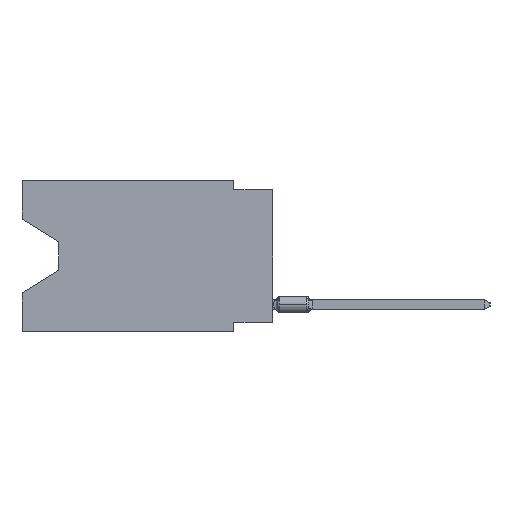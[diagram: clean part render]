
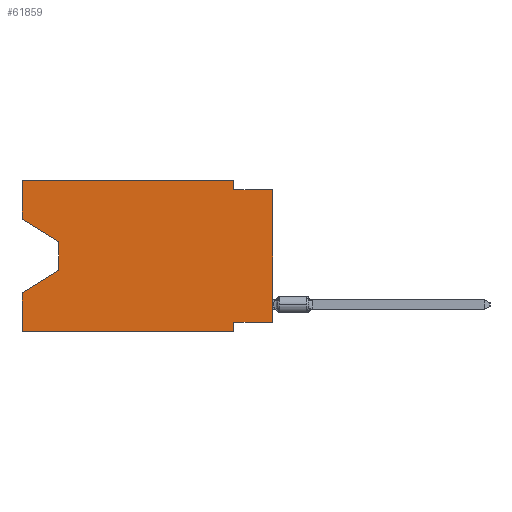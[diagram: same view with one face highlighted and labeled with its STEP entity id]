
A CAD part, left-side view. The second image highlights one B-rep face of the part: STEP entity #61859.
In plain terms, the highlighted planar face has unit normal (-1, 0, 0).
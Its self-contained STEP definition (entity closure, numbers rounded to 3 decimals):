
#145 = DIRECTION ( 'NONE',  ( 0., -1., 0. ) ) ;
#579 = VECTOR ( 'NONE', #29271, 1000. ) ;
#1205 = ORIENTED_EDGE ( 'NONE', *, *, #51007, .F. ) ;
#2809 = VECTOR ( 'NONE', #14306, 1000. ) ;
#3244 = VECTOR ( 'NONE', #65804, 1000. ) ;
#4586 = EDGE_CURVE ( 'NONE', #47050, #57609, #53445, .T. ) ;
#6383 = CARTESIAN_POINT ( 'NONE',  ( 0., 16.383, -2.546 ) ) ;
#7798 = DIRECTION ( 'NONE',  ( 0., 0., -1. ) ) ;
#8413 = DIRECTION ( 'NONE',  ( 0., 0., -1. ) ) ;
#9014 = LINE ( 'NONE', #40310, #3244 ) ;
#10100 = VERTEX_POINT ( 'NONE', #64654 ) ;
#10206 = VECTOR ( 'NONE', #25276, 1000. ) ;
#10544 = LINE ( 'NONE', #61910, #56642 ) ;
#11691 = ORIENTED_EDGE ( 'NONE', *, *, #68116, .F. ) ;
#11780 = DIRECTION ( 'NONE',  ( 0., 0., 1. ) ) ;
#12671 = VECTOR ( 'NONE', #71596, 1000. ) ;
#13353 = VERTEX_POINT ( 'NONE', #50431 ) ;
#14019 = CARTESIAN_POINT ( 'NONE',  ( 0., 0., -9.271 ) ) ;
#14274 = LINE ( 'NONE', #78240, #31240 ) ;
#14306 = DIRECTION ( 'NONE',  ( 0., -1., 0. ) ) ;
#15611 = VERTEX_POINT ( 'NONE', #37214 ) ;
#16272 = DIRECTION ( 'NONE',  ( 0., -0.855, -0.519 ) ) ;
#16554 = ORIENTED_EDGE ( 'NONE', *, *, #73039, .F. ) ;
#18829 = AXIS2_PLACEMENT_3D ( 'NONE', #31843, #76595, #69478 ) ;
#19768 = LINE ( 'NONE', #59008, #12671 ) ;
#19928 = CARTESIAN_POINT ( 'NONE',  ( 0., 2.54, 0. ) ) ;
#20248 = DIRECTION ( 'NONE',  ( 0., 0., 1. ) ) ;
#23262 = DIRECTION ( 'NONE',  ( 0., 0., -1. ) ) ;
#24398 = CARTESIAN_POINT ( 'NONE',  ( 0., 13.97, -5.893 ) ) ;
#25230 = CARTESIAN_POINT ( 'NONE',  ( 0., 16.383, 0. ) ) ;
#25265 = EDGE_CURVE ( 'NONE', #73610, #44479, #14274, .T. ) ;
#25276 = DIRECTION ( 'NONE',  ( 0., 0., 1. ) ) ;
#26128 = LINE ( 'NONE', #40711, #39667 ) ;
#29271 = DIRECTION ( 'NONE',  ( 0., 1., 0. ) ) ;
#29768 = VERTEX_POINT ( 'NONE', #14019 ) ;
#29986 = EDGE_CURVE ( 'NONE', #54463, #15611, #9014, .T. ) ;
#31240 = VECTOR ( 'NONE', #8413, 1000. ) ;
#31843 = CARTESIAN_POINT ( 'NONE',  ( 0., 16.383, 0. ) ) ;
#32245 = PLANE ( 'NONE',  #18829 ) ;
#32410 = VECTOR ( 'NONE', #16272, 1000. ) ;
#33087 = LINE ( 'NONE', #40595, #2809 ) ;
#33813 = CARTESIAN_POINT ( 'NONE',  ( 0., 16.383, -2.546 ) ) ;
#35111 = CARTESIAN_POINT ( 'NONE',  ( 0., 0., -9.271 ) ) ;
#37214 = CARTESIAN_POINT ( 'NONE',  ( 0., 16.383, -7.36 ) ) ;
#38207 = CARTESIAN_POINT ( 'NONE',  ( 0., 16.383, 0. ) ) ;
#38566 = LINE ( 'NONE', #25230, #77354 ) ;
#38640 = CARTESIAN_POINT ( 'NONE',  ( 0., 2.54, -0.635 ) ) ;
#39459 = LINE ( 'NONE', #38207, #10206 ) ;
#39527 = LINE ( 'NONE', #75943, #71378 ) ;
#39667 = VECTOR ( 'NONE', #20248, 1000. ) ;
#40310 = CARTESIAN_POINT ( 'NONE',  ( 0., 13.97, -5.893 ) ) ;
#40595 = CARTESIAN_POINT ( 'NONE',  ( 0., 16.383, -9.906 ) ) ;
#40711 = CARTESIAN_POINT ( 'NONE',  ( 0., 0., 0. ) ) ;
#42141 = ORIENTED_EDGE ( 'NONE', *, *, #55748, .T. ) ;
#42194 = VERTEX_POINT ( 'NONE', #82650 ) ;
#43062 = VERTEX_POINT ( 'NONE', #62137 ) ;
#43929 = CARTESIAN_POINT ( 'NONE',  ( 0., 13.97, -4.013 ) ) ;
#44479 = VERTEX_POINT ( 'NONE', #38640 ) ;
#46908 = ORIENTED_EDGE ( 'NONE', *, *, #53193, .F. ) ;
#47050 = VERTEX_POINT ( 'NONE', #6383 ) ;
#47084 = CARTESIAN_POINT ( 'NONE',  ( 0., 13.97, -4.013 ) ) ;
#50431 = CARTESIAN_POINT ( 'NONE',  ( 0., 2.54, -9.271 ) ) ;
#51007 = EDGE_CURVE ( 'NONE', #43062, #15611, #10544, .T. ) ;
#53193 = EDGE_CURVE ( 'NONE', #13353, #42194, #39527, .T. ) ;
#53445 = LINE ( 'NONE', #33813, #32410 ) ;
#53508 = ORIENTED_EDGE ( 'NONE', *, *, #29986, .T. ) ;
#53751 = LINE ( 'NONE', #47084, #64881 ) ;
#53772 = ORIENTED_EDGE ( 'NONE', *, *, #81179, .F. ) ;
#54463 = VERTEX_POINT ( 'NONE', #24398 ) ;
#55499 = ORIENTED_EDGE ( 'NONE', *, *, #77232, .F. ) ;
#55748 = EDGE_CURVE ( 'NONE', #29768, #10100, #26128, .T. ) ;
#56642 = VECTOR ( 'NONE', #11780, 1000. ) ;
#57609 = VERTEX_POINT ( 'NONE', #43929 ) ;
#59008 = CARTESIAN_POINT ( 'NONE',  ( 0., 0., -0.635 ) ) ;
#60697 = ORIENTED_EDGE ( 'NONE', *, *, #61984, .T. ) ;
#61444 = LINE ( 'NONE', #35111, #579 ) ;
#61859 = ADVANCED_FACE ( 'NONE', ( #64435 ), #32245, .F. ) ;
#61910 = CARTESIAN_POINT ( 'NONE',  ( 0., 16.383, 0. ) ) ;
#61984 = EDGE_CURVE ( 'NONE', #43062, #42194, #33087, .T. ) ;
#62137 = CARTESIAN_POINT ( 'NONE',  ( 0., 16.383, -9.906 ) ) ;
#62874 = EDGE_LOOP ( 'NONE', ( #67131, #80771, #53508, #1205, #60697, #46908, #16554, #42141, #11691, #66356, #53772, #55499 ) ) ;
#64435 = FACE_OUTER_BOUND ( 'NONE', #62874, .T. ) ;
#64654 = CARTESIAN_POINT ( 'NONE',  ( 0., 0., -0.635 ) ) ;
#64881 = VECTOR ( 'NONE', #23262, 1000. ) ;
#65804 = DIRECTION ( 'NONE',  ( 0., 0.855, -0.519 ) ) ;
#66356 = ORIENTED_EDGE ( 'NONE', *, *, #25265, .F. ) ;
#67046 = CARTESIAN_POINT ( 'NONE',  ( 0., 16.383, 0. ) ) ;
#67131 = ORIENTED_EDGE ( 'NONE', *, *, #4586, .T. ) ;
#67453 = EDGE_CURVE ( 'NONE', #57609, #54463, #53751, .T. ) ;
#68116 = EDGE_CURVE ( 'NONE', #44479, #10100, #19768, .T. ) ;
#69025 = VERTEX_POINT ( 'NONE', #67046 ) ;
#69478 = DIRECTION ( 'NONE',  ( 0., 0., -1. ) ) ;
#71378 = VECTOR ( 'NONE', #7798, 1000. ) ;
#71596 = DIRECTION ( 'NONE',  ( 0., -1., 0. ) ) ;
#73039 = EDGE_CURVE ( 'NONE', #29768, #13353, #61444, .T. ) ;
#73610 = VERTEX_POINT ( 'NONE', #19928 ) ;
#75943 = CARTESIAN_POINT ( 'NONE',  ( 0., 2.54, -9.906 ) ) ;
#76595 = DIRECTION ( 'NONE',  ( 1., 0., 0. ) ) ;
#77232 = EDGE_CURVE ( 'NONE', #47050, #69025, #39459, .T. ) ;
#77354 = VECTOR ( 'NONE', #145, 1000. ) ;
#78240 = CARTESIAN_POINT ( 'NONE',  ( 0., 2.54, 0. ) ) ;
#80771 = ORIENTED_EDGE ( 'NONE', *, *, #67453, .T. ) ;
#81179 = EDGE_CURVE ( 'NONE', #69025, #73610, #38566, .T. ) ;
#82650 = CARTESIAN_POINT ( 'NONE',  ( 0., 2.54, -9.906 ) ) ;
